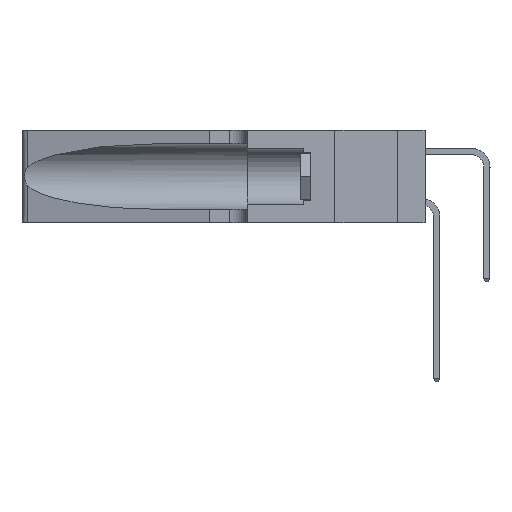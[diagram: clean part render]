
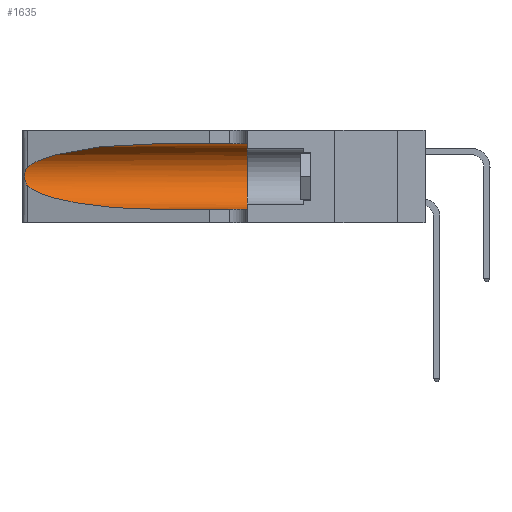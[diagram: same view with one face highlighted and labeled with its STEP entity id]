
A CAD part, left-side view. The second image highlights one B-rep face of the part: STEP entity #1635.
In plain terms, the highlighted cylindrical face has radius 3.308 mm (diameter 6.617 mm), a partial arc.
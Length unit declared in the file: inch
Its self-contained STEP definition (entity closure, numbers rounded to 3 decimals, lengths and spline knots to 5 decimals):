
#1635 = ADVANCED_FACE ( 'NONE', ( #26407 ), #19272, .F. ) ;
#1686 = DIRECTION ( 'NONE',  ( 0., -1., 0. ) ) ;
#1758 = CARTESIAN_POINT ( 'NONE',  ( 0.25555, 1.22993, 0.14849 ) ) ;
#1943 = VERTEX_POINT ( 'NONE', #30577 ) ;
#2068 = VECTOR ( 'NONE', #1686, 39.37008 ) ;
#2881 = ORIENTED_EDGE ( 'NONE', *, *, #12913, .F. ) ;
#3234 = EDGE_LOOP ( 'NONE', ( #19219, #6075, #19724, #20244, #2881, #30868 ) ) ;
#4419 = CARTESIAN_POINT ( 'NONE',  ( 0.25639, 1.23184, 0.21858 ) ) ;
#4489 = EDGE_CURVE ( 'NONE', #1943, #18175, #30805, .T. ) ;
#4532 = VERTEX_POINT ( 'NONE', #34241 ) ;
#4540 = CARTESIAN_POINT ( 'NONE',  ( 0.18966, 0.96281, 0.31525 ) ) ;
#5133 = EDGE_CURVE ( 'NONE', #28394, #32541, #34519, .T. ) ;
#5155 = EDGE_CURVE ( 'NONE', #4532, #28394, #28335, .T. ) ;
#6075 = ORIENTED_EDGE ( 'NONE', *, *, #5133, .T. ) ;
#6406 = EDGE_CURVE ( 'NONE', #4532, #33496, #8883, .T. ) ;
#7219 = CARTESIAN_POINT ( 'NONE',  ( 0.25787, 1.23484, 0.2124 ) ) ;
#8502 = CARTESIAN_POINT ( 'NONE',  ( 0.25487, 1.22718, 0.22369 ) ) ;
#8801 = CARTESIAN_POINT ( 'NONE',  ( 0.2373, 1.15595, 0.08982 ) ) ;
#8883 = LINE ( 'NONE', #20807, #14355 ) ;
#9937 = CARTESIAN_POINT ( 'NONE',  ( 0.26018, 1.23835, 0.19895 ) ) ;
#10350 = CARTESIAN_POINT ( 'NONE',  ( 0.1305, 0.35, 0.31525 ) ) ;
#10525 = CARTESIAN_POINT ( 'NONE',  ( 0.1305, 1.61858, 0.185 ) ) ;
#11495 = CARTESIAN_POINT ( 'NONE',  ( 0.18966, 0.96281, 0.05475 ) ) ;
#12645 = CARTESIAN_POINT ( 'NONE',  ( 0.26075, 1.23896, 0.178 ) ) ;
#12757 = CARTESIAN_POINT ( 'NONE',  ( 0.25487, 1.22718, 0.22369 ) ) ;
#12913 = EDGE_CURVE ( 'NONE', #33496, #18175, #22622, .T. ) ;
#14355 = VECTOR ( 'NONE', #18085, 39.37008 ) ;
#15012 = CARTESIAN_POINT ( 'NONE',  ( 0.1305, 0.35, 0.185 ) ) ;
#15222 = CARTESIAN_POINT ( 'NONE',  ( 0.25555, 1.22994, 0.2215 ) ) ;
#15341 = CARTESIAN_POINT ( 'NONE',  ( 0.25856, 1.23593, 0.16098 ) ) ;
#17443 = CARTESIAN_POINT ( 'NONE',  ( 0.25487, 1.22718, 0.14631 ) ) ;
#17713 = DIRECTION ( 'NONE',  ( 0., 0., 1. ) ) ;
#17845 = CARTESIAN_POINT ( 'NONE',  ( 0.1305, 1.61858, 0.05475 ) ) ;
#17916 = CARTESIAN_POINT ( 'NONE',  ( 0.1305, 0.72297, 0.31525 ) ) ;
#18044 = CARTESIAN_POINT ( 'NONE',  ( 0.25639, 1.23186, 0.15144 ) ) ;
#18085 = DIRECTION ( 'NONE',  ( 0., -1., 0. ) ) ;
#18175 = VERTEX_POINT ( 'NONE', #24765 ) ;
#19118 = EDGE_CURVE ( 'NONE', #32541, #1943, #25748, .T. ) ;
#19219 = ORIENTED_EDGE ( 'NONE', *, *, #5155, .T. ) ;
#19272 = CYLINDRICAL_SURFACE ( 'NONE', #20930, 0.13025 ) ;
#19724 = ORIENTED_EDGE ( 'NONE', *, *, #19118, .T. ) ;
#20244 = ORIENTED_EDGE ( 'NONE', *, *, #4489, .T. ) ;
#20755 = CARTESIAN_POINT ( 'NONE',  ( 0.25487, 1.22718, 0.14631 ) ) ;
#20807 = CARTESIAN_POINT ( 'NONE',  ( 0.1305, 1.61858, 0.31525 ) ) ;
#20930 = AXIS2_PLACEMENT_3D ( 'NONE', #10525, #21338, #24056 ) ;
#21338 = DIRECTION ( 'NONE',  ( 0., -1., 0. ) ) ;
#22622 = CIRCLE ( 'NONE', #29034, 0.13025 ) ;
#23245 = CARTESIAN_POINT ( 'NONE',  ( 0.25487, 1.22718, 0.22369 ) ) ;
#24056 = DIRECTION ( 'NONE',  ( 0., 0., -1. ) ) ;
#24765 = CARTESIAN_POINT ( 'NONE',  ( 0.1305, 0.35, 0.05475 ) ) ;
#24897 = CARTESIAN_POINT ( 'NONE',  ( 0.25487, 1.22718, 0.14631 ) ) ;
#25748 =( BOUNDED_CURVE ( )  B_SPLINE_CURVE ( 3, ( #24897, #8801, #11495, #30272 ),
 .UNSPECIFIED., .F., .T. ) 
 B_SPLINE_CURVE_WITH_KNOTS ( ( 4, 4 ),
 ( 3.44316, 4.71239 ),
 .UNSPECIFIED. ) 
 CURVE ( )  GEOMETRIC_REPRESENTATION_ITEM ( )  RATIONAL_B_SPLINE_CURVE ( ( 1., 0.87, 0.87, 1. ) ) 
 REPRESENTATION_ITEM ( '' )  );
#26036 = CARTESIAN_POINT ( 'NONE',  ( 0.25854, 1.2359, 0.20912 ) ) ;
#26407 = FACE_OUTER_BOUND ( 'NONE', #3234, .T. ) ;
#28335 =( BOUNDED_CURVE ( )  B_SPLINE_CURVE ( 3, ( #17916, #4540, #28857, #12757 ),
 .UNSPECIFIED., .F., .F. ) 
 B_SPLINE_CURVE_WITH_KNOTS ( ( 4, 4 ),
 ( 1.5708, 2.84003 ),
 .UNSPECIFIED. ) 
 CURVE ( )  GEOMETRIC_REPRESENTATION_ITEM ( )  RATIONAL_B_SPLINE_CURVE ( ( 1., 0.87, 0.87, 1. ) ) 
 REPRESENTATION_ITEM ( '' )  );
#28394 = VERTEX_POINT ( 'NONE', #8502 ) ;
#28731 = CARTESIAN_POINT ( 'NONE',  ( 0.26075, 1.23896, 0.19203 ) ) ;
#28857 = CARTESIAN_POINT ( 'NONE',  ( 0.2373, 1.15595, 0.28018 ) ) ;
#29034 = AXIS2_PLACEMENT_3D ( 'NONE', #15012, #33771, #17713 ) ;
#30272 = CARTESIAN_POINT ( 'NONE',  ( 0.1305, 0.72297, 0.05475 ) ) ;
#30577 = CARTESIAN_POINT ( 'NONE',  ( 0.1305, 0.72297, 0.05475 ) ) ;
#30805 = LINE ( 'NONE', #17845, #2068 ) ;
#30868 = ORIENTED_EDGE ( 'NONE', *, *, #6406, .F. ) ;
#31405 = CARTESIAN_POINT ( 'NONE',  ( 0.26017, 1.23833, 0.17102 ) ) ;
#32541 = VERTEX_POINT ( 'NONE', #17443 ) ;
#33496 = VERTEX_POINT ( 'NONE', #10350 ) ;
#33771 = DIRECTION ( 'NONE',  ( 0., 1., 0. ) ) ;
#34084 = CARTESIAN_POINT ( 'NONE',  ( 0.25789, 1.23486, 0.15765 ) ) ;
#34241 = CARTESIAN_POINT ( 'NONE',  ( 0.1305, 0.72297, 0.31525 ) ) ;
#34519 = B_SPLINE_CURVE_WITH_KNOTS ( 'NONE', 3,
 ( #23245, #15222, #4419, #7219, #26036, #9937, #28731, #12645, #31405, #15341, #34084, #18044, #1758, #20755 ),
 .UNSPECIFIED., .F., .F.,
 ( 4, 2, 2, 2, 2, 2, 4 ),
 ( 0., 0.00027, 0.00053, 0.00107, 0.0016, 0.00187, 0.00214 ),
 .UNSPECIFIED. ) ;
